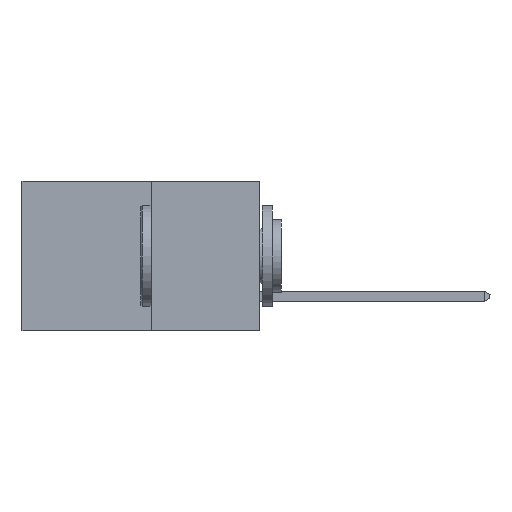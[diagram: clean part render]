
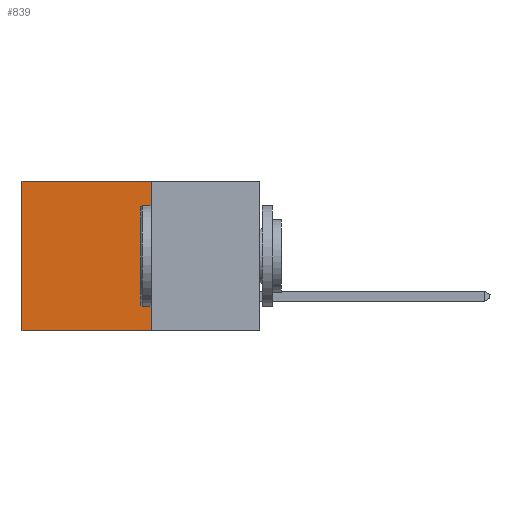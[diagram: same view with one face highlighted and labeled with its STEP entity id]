
A CAD part, left-side view. The second image highlights one B-rep face of the part: STEP entity #839.
In plain terms, the highlighted planar face has unit normal (-1, 0, 0).
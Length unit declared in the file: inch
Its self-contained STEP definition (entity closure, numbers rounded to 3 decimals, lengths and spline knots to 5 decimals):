
#131 = FACE_OUTER_BOUND ( 'NONE', #23413, .T. ) ;
#326 = LINE ( 'NONE', #9196, #17618 ) ;
#839 = ADVANCED_FACE ( 'NONE', ( #131 ), #2857, .F. ) ;
#1484 = VECTOR ( 'NONE', #3462, 39.37008 ) ;
#1857 = CARTESIAN_POINT ( 'NONE',  ( 0.277, 0.27, -0.37 ) ) ;
#2202 = LINE ( 'NONE', #17902, #1484 ) ;
#2578 = LINE ( 'NONE', #11998, #25787 ) ;
#2593 = EDGE_CURVE ( 'NONE', #4233, #12072, #2202, .T. ) ;
#2857 = PLANE ( 'NONE',  #13403 ) ;
#3445 = DIRECTION ( 'NONE',  ( 0., 0., -1. ) ) ;
#3462 = DIRECTION ( 'NONE',  ( 0., 0., -1. ) ) ;
#4233 = VERTEX_POINT ( 'NONE', #13902 ) ;
#7680 = DIRECTION ( 'NONE',  ( 0., 1., 0. ) ) ;
#9196 = CARTESIAN_POINT ( 'NONE',  ( 0.277, 0.27, 0. ) ) ;
#9703 = ORIENTED_EDGE ( 'NONE', *, *, #22846, .T. ) ;
#11463 = DIRECTION ( 'NONE',  ( 0., 1., 0. ) ) ;
#11493 = EDGE_CURVE ( 'NONE', #12072, #22962, #12208, .T. ) ;
#11500 = VECTOR ( 'NONE', #7680, 39.37008 ) ;
#11998 = CARTESIAN_POINT ( 'NONE',  ( 0.277, 0.59, -0.37 ) ) ;
#12002 = EDGE_CURVE ( 'NONE', #24724, #22962, #2578, .T. ) ;
#12072 = VERTEX_POINT ( 'NONE', #21391 ) ;
#12208 = LINE ( 'NONE', #18732, #11500 ) ;
#13403 = AXIS2_PLACEMENT_3D ( 'NONE', #1857, #28736, #17637 ) ;
#13902 = CARTESIAN_POINT ( 'NONE',  ( 0.277, 0.27, 0. ) ) ;
#17618 = VECTOR ( 'NONE', #11463, 39.37008 ) ;
#17637 = DIRECTION ( 'NONE',  ( 0., 0., -1. ) ) ;
#17902 = CARTESIAN_POINT ( 'NONE',  ( 0.277, 0.27, -0.37 ) ) ;
#18732 = CARTESIAN_POINT ( 'NONE',  ( 0.277, 0.27, -0.37 ) ) ;
#20244 = CARTESIAN_POINT ( 'NONE',  ( 0.277, 0.59, 0. ) ) ;
#21391 = CARTESIAN_POINT ( 'NONE',  ( 0.277, 0.27, -0.37 ) ) ;
#21684 = ORIENTED_EDGE ( 'NONE', *, *, #12002, .T. ) ;
#22037 = ORIENTED_EDGE ( 'NONE', *, *, #2593, .F. ) ;
#22846 = EDGE_CURVE ( 'NONE', #4233, #24724, #326, .T. ) ;
#22962 = VERTEX_POINT ( 'NONE', #25098 ) ;
#23413 = EDGE_LOOP ( 'NONE', ( #21684, #25296, #22037, #9703 ) ) ;
#24724 = VERTEX_POINT ( 'NONE', #20244 ) ;
#25098 = CARTESIAN_POINT ( 'NONE',  ( 0.277, 0.59, -0.37 ) ) ;
#25296 = ORIENTED_EDGE ( 'NONE', *, *, #11493, .F. ) ;
#25787 = VECTOR ( 'NONE', #3445, 39.37008 ) ;
#28736 = DIRECTION ( 'NONE',  ( 1., 0., 0. ) ) ;
